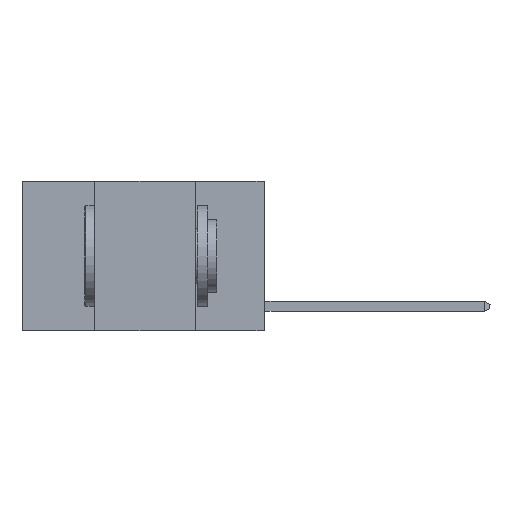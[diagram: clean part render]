
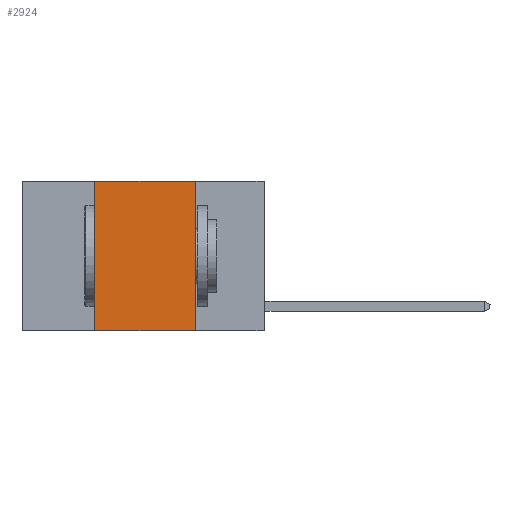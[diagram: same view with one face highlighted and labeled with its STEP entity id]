
A CAD part, left-side view. The second image highlights one B-rep face of the part: STEP entity #2924.
In plain terms, the highlighted planar face has unit normal (-1, 0, 0).
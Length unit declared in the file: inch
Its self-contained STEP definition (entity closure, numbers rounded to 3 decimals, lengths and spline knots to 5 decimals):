
#223 = EDGE_CURVE ( 'NONE', #1334, #10237, #13955, .T. ) ;
#1071 = VERTEX_POINT ( 'NONE', #13907 ) ;
#1113 = LINE ( 'NONE', #19431, #11511 ) ;
#1334 = VERTEX_POINT ( 'NONE', #23176 ) ;
#2924 = ADVANCED_FACE ( 'NONE', ( #7788 ), #16858, .F. ) ;
#3018 = VECTOR ( 'NONE', #18825, 39.37008 ) ;
#3306 = CARTESIAN_POINT ( 'NONE',  ( 0., 0.6, 0. ) ) ;
#4544 = ORIENTED_EDGE ( 'NONE', *, *, #16345, .T. ) ;
#5623 = DIRECTION ( 'NONE',  ( 0., -1., 0. ) ) ;
#6097 = CARTESIAN_POINT ( 'NONE',  ( 0., 0.6, -0.37 ) ) ;
#7788 = FACE_OUTER_BOUND ( 'NONE', #19693, .T. ) ;
#8045 = DIRECTION ( 'NONE',  ( 0., -1., 0. ) ) ;
#8848 = CARTESIAN_POINT ( 'NONE',  ( 0., 0.42, 0. ) ) ;
#10237 = VERTEX_POINT ( 'NONE', #14740 ) ;
#10688 = AXIS2_PLACEMENT_3D ( 'NONE', #3306, #11176, #24475 ) ;
#11069 = LINE ( 'NONE', #15237, #15566 ) ;
#11118 = ORIENTED_EDGE ( 'NONE', *, *, #15019, .F. ) ;
#11176 = DIRECTION ( 'NONE',  ( 1., 0., 0. ) ) ;
#11185 = CARTESIAN_POINT ( 'NONE',  ( 0., 0.17, 0. ) ) ;
#11511 = VECTOR ( 'NONE', #15605, 39.37008 ) ;
#13296 = ORIENTED_EDGE ( 'NONE', *, *, #17446, .F. ) ;
#13907 = CARTESIAN_POINT ( 'NONE',  ( 0., 0.42, -0.37 ) ) ;
#13955 = LINE ( 'NONE', #11185, #3018 ) ;
#14740 = CARTESIAN_POINT ( 'NONE',  ( 0., 0.17, -0.37 ) ) ;
#15019 = EDGE_CURVE ( 'NONE', #1071, #22435, #1113, .T. ) ;
#15237 = CARTESIAN_POINT ( 'NONE',  ( 0., 0.6, 0. ) ) ;
#15566 = VECTOR ( 'NONE', #5623, 39.37008 ) ;
#15605 = DIRECTION ( 'NONE',  ( 0., 0., 1. ) ) ;
#16345 = EDGE_CURVE ( 'NONE', #1071, #10237, #17116, .T. ) ;
#16858 = PLANE ( 'NONE',  #10688 ) ;
#17116 = LINE ( 'NONE', #6097, #17704 ) ;
#17446 = EDGE_CURVE ( 'NONE', #22435, #1334, #11069, .T. ) ;
#17704 = VECTOR ( 'NONE', #8045, 39.37008 ) ;
#18825 = DIRECTION ( 'NONE',  ( 0., 0., -1. ) ) ;
#19431 = CARTESIAN_POINT ( 'NONE',  ( 0., 0.42, 0. ) ) ;
#19693 = EDGE_LOOP ( 'NONE', ( #24500, #13296, #11118, #4544 ) ) ;
#22435 = VERTEX_POINT ( 'NONE', #8848 ) ;
#23176 = CARTESIAN_POINT ( 'NONE',  ( 0., 0.17, 0. ) ) ;
#24475 = DIRECTION ( 'NONE',  ( 0., 0., -1. ) ) ;
#24500 = ORIENTED_EDGE ( 'NONE', *, *, #223, .F. ) ;
